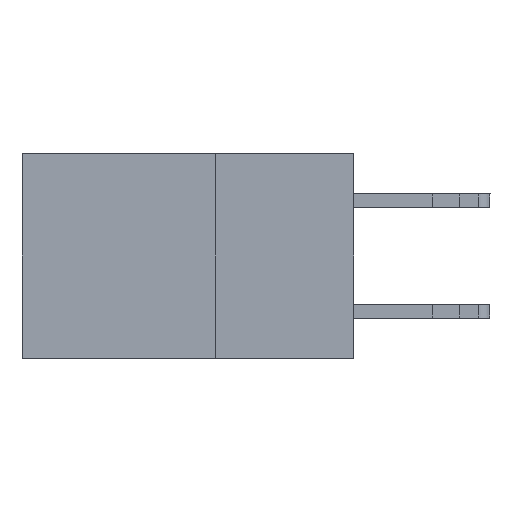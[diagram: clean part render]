
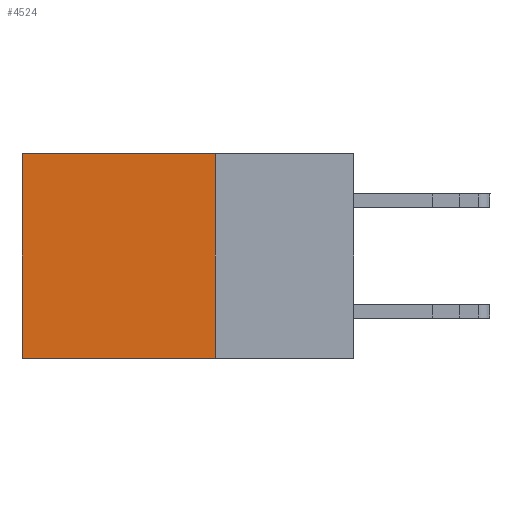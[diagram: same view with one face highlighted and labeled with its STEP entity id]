
A CAD part, left-side view. The second image highlights one B-rep face of the part: STEP entity #4524.
In plain terms, the highlighted planar face has unit normal (-1, 0, 0).
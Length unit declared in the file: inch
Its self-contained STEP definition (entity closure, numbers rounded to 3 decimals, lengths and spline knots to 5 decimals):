
#323 = VECTOR ( 'NONE', #6344, 39.37008 ) ;
#3439 = VECTOR ( 'NONE', #23212, 39.37008 ) ;
#3535 = DIRECTION ( 'NONE',  ( 0., 0., -1. ) ) ;
#4524 = ADVANCED_FACE ( 'NONE', ( #35172 ), #26466, .F. ) ;
#4786 = CARTESIAN_POINT ( 'NONE',  ( 0.2875, 0.25, 0. ) ) ;
#6344 = DIRECTION ( 'NONE',  ( 0., 0., -1. ) ) ;
#8835 = LINE ( 'NONE', #18438, #323 ) ;
#9929 = CARTESIAN_POINT ( 'NONE',  ( 0.2875, 0.25, -0.37 ) ) ;
#10195 = ORIENTED_EDGE ( 'NONE', *, *, #28798, .F. ) ;
#10648 = EDGE_LOOP ( 'NONE', ( #15637, #13066, #10195, #34735 ) ) ;
#10738 = CARTESIAN_POINT ( 'NONE',  ( 0.2875, 0.25, -0.37 ) ) ;
#11972 = EDGE_CURVE ( 'NONE', #31510, #37520, #28287, .T. ) ;
#12982 = EDGE_CURVE ( 'NONE', #20160, #37520, #23532, .T. ) ;
#13066 = ORIENTED_EDGE ( 'NONE', *, *, #11972, .F. ) ;
#14231 = VECTOR ( 'NONE', #22677, 39.37008 ) ;
#15393 = DIRECTION ( 'NONE',  ( 1., 0., 0. ) ) ;
#15637 = ORIENTED_EDGE ( 'NONE', *, *, #12982, .T. ) ;
#16085 = CARTESIAN_POINT ( 'NONE',  ( 0.2875, 0.6, -0.37 ) ) ;
#16349 = CARTESIAN_POINT ( 'NONE',  ( 0.2875, 0.6, 0. ) ) ;
#16961 = VECTOR ( 'NONE', #28384, 39.37008 ) ;
#18438 = CARTESIAN_POINT ( 'NONE',  ( 0.2875, 0.25, 0. ) ) ;
#20109 = VERTEX_POINT ( 'NONE', #4786 ) ;
#20160 = VERTEX_POINT ( 'NONE', #37440 ) ;
#22677 = DIRECTION ( 'NONE',  ( 0., 1., 0. ) ) ;
#23212 = DIRECTION ( 'NONE',  ( 0., 1., 0. ) ) ;
#23532 = LINE ( 'NONE', #16349, #16961 ) ;
#24506 = AXIS2_PLACEMENT_3D ( 'NONE', #29432, #15393, #3535 ) ;
#26394 = LINE ( 'NONE', #37916, #3439 ) ;
#26466 = PLANE ( 'NONE',  #24506 ) ;
#28287 = LINE ( 'NONE', #9929, #14231 ) ;
#28384 = DIRECTION ( 'NONE',  ( 0., 0., -1. ) ) ;
#28798 = EDGE_CURVE ( 'NONE', #20109, #31510, #8835, .T. ) ;
#29432 = CARTESIAN_POINT ( 'NONE',  ( 0.2875, 0.25, 0. ) ) ;
#31510 = VERTEX_POINT ( 'NONE', #10738 ) ;
#33105 = EDGE_CURVE ( 'NONE', #20109, #20160, #26394, .T. ) ;
#34735 = ORIENTED_EDGE ( 'NONE', *, *, #33105, .T. ) ;
#35172 = FACE_OUTER_BOUND ( 'NONE', #10648, .T. ) ;
#37440 = CARTESIAN_POINT ( 'NONE',  ( 0.2875, 0.6, 0. ) ) ;
#37520 = VERTEX_POINT ( 'NONE', #16085 ) ;
#37916 = CARTESIAN_POINT ( 'NONE',  ( 0.2875, 0.25, 0. ) ) ;
